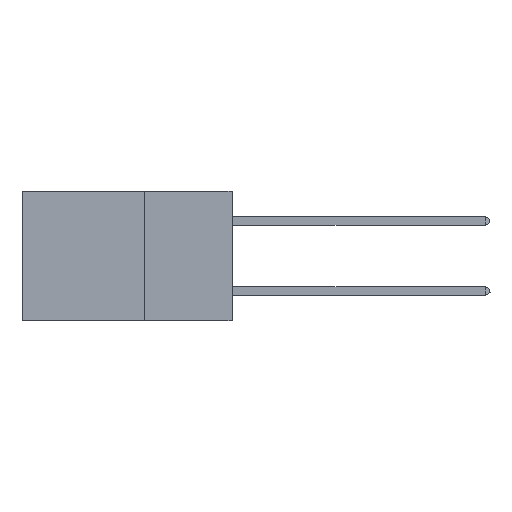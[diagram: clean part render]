
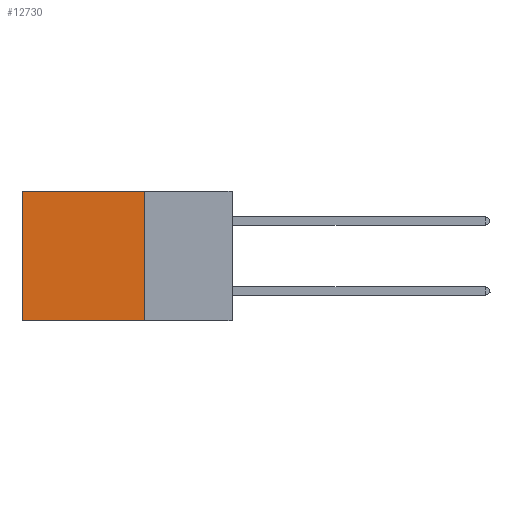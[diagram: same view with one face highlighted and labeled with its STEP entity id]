
A CAD part, left-side view. The second image highlights one B-rep face of the part: STEP entity #12730.
In plain terms, the highlighted planar face has unit normal (-1, 0, 0).
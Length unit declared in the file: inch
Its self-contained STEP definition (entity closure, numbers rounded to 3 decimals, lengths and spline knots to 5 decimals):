
#291 = VERTEX_POINT ( 'NONE', #15288 ) ;
#1127 = ORIENTED_EDGE ( 'NONE', *, *, #4565, .F. ) ;
#1670 = FACE_OUTER_BOUND ( 'NONE', #19233, .T. ) ;
#1713 = CARTESIAN_POINT ( 'NONE',  ( 0.2875, 0.25, 0. ) ) ;
#1953 = VERTEX_POINT ( 'NONE', #2142 ) ;
#2142 = CARTESIAN_POINT ( 'NONE',  ( 0.2875, 0.25, -0.37 ) ) ;
#2194 = VECTOR ( 'NONE', #9176, 39.37008 ) ;
#2695 = LINE ( 'NONE', #22285, #11107 ) ;
#2910 = ORIENTED_EDGE ( 'NONE', *, *, #19984, .F. ) ;
#4565 = EDGE_CURVE ( 'NONE', #1953, #13275, #2695, .T. ) ;
#9176 = DIRECTION ( 'NONE',  ( 0., 1., 0. ) ) ;
#10294 = AXIS2_PLACEMENT_3D ( 'NONE', #37828, #28388, #31591 ) ;
#11107 = VECTOR ( 'NONE', #32284, 39.37008 ) ;
#12730 = ADVANCED_FACE ( 'NONE', ( #1670 ), #24788, .F. ) ;
#13275 = VERTEX_POINT ( 'NONE', #30982 ) ;
#15288 = CARTESIAN_POINT ( 'NONE',  ( 0.2875, 0.25, 0. ) ) ;
#15676 = EDGE_CURVE ( 'NONE', #291, #27697, #38953, .T. ) ;
#16556 = DIRECTION ( 'NONE',  ( 0., 0., -1. ) ) ;
#19233 = EDGE_LOOP ( 'NONE', ( #41105, #1127, #2910, #20613 ) ) ;
#19984 = EDGE_CURVE ( 'NONE', #291, #1953, #25214, .T. ) ;
#20613 = ORIENTED_EDGE ( 'NONE', *, *, #15676, .T. ) ;
#22285 = CARTESIAN_POINT ( 'NONE',  ( 0.2875, 0.25, -0.37 ) ) ;
#23727 = VECTOR ( 'NONE', #23912, 39.37008 ) ;
#23912 = DIRECTION ( 'NONE',  ( 0., 0., -1. ) ) ;
#24788 = PLANE ( 'NONE',  #10294 ) ;
#25214 = LINE ( 'NONE', #1713, #23727 ) ;
#27697 = VERTEX_POINT ( 'NONE', #35462 ) ;
#28388 = DIRECTION ( 'NONE',  ( 1., 0., 0. ) ) ;
#30356 = EDGE_CURVE ( 'NONE', #27697, #13275, #40461, .T. ) ;
#30982 = CARTESIAN_POINT ( 'NONE',  ( 0.2875, 0.6, -0.37 ) ) ;
#31591 = DIRECTION ( 'NONE',  ( 0., 0., -1. ) ) ;
#32284 = DIRECTION ( 'NONE',  ( 0., 1., 0. ) ) ;
#33013 = VECTOR ( 'NONE', #16556, 39.37008 ) ;
#35462 = CARTESIAN_POINT ( 'NONE',  ( 0.2875, 0.6, 0. ) ) ;
#37828 = CARTESIAN_POINT ( 'NONE',  ( 0.2875, 0.25, 0. ) ) ;
#38871 = CARTESIAN_POINT ( 'NONE',  ( 0.2875, 0.6, 0. ) ) ;
#38953 = LINE ( 'NONE', #40820, #2194 ) ;
#40461 = LINE ( 'NONE', #38871, #33013 ) ;
#40820 = CARTESIAN_POINT ( 'NONE',  ( 0.2875, 0.25, 0. ) ) ;
#41105 = ORIENTED_EDGE ( 'NONE', *, *, #30356, .T. ) ;
